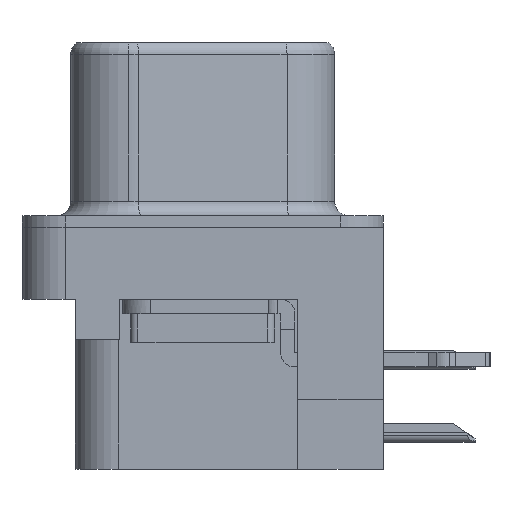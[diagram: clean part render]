
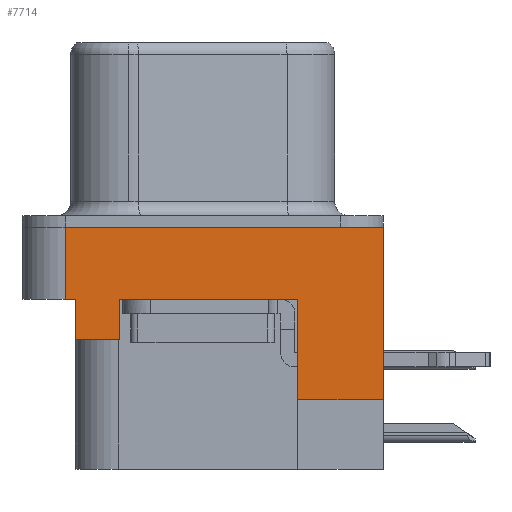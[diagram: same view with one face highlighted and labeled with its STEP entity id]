
A CAD part, left-side view. The second image highlights one B-rep face of the part: STEP entity #7714.
In plain terms, the highlighted planar face has unit normal (-1, 0, 0).
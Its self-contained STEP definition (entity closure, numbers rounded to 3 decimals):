
#115 = CARTESIAN_POINT ( 'NONE',  ( -3., -3.295, -6. ) ) ;
#613 = CARTESIAN_POINT ( 'NONE',  ( -3., 4.425, -3.9 ) ) ;
#843 = VECTOR ( 'NONE', #7435, 1000. ) ;
#917 = AXIS2_PLACEMENT_3D ( 'NONE', #3185, #8487, #19113 ) ;
#1014 = ORIENTED_EDGE ( 'NONE', *, *, #11626, .F. ) ;
#1609 = VECTOR ( 'NONE', #16953, 1000. ) ;
#1966 = VERTEX_POINT ( 'NONE', #12469 ) ;
#2138 = VERTEX_POINT ( 'NONE', #115 ) ;
#3038 = VERTEX_POINT ( 'NONE', #7005 ) ;
#3185 = CARTESIAN_POINT ( 'NONE',  ( -3., -6.275, -2.5 ) ) ;
#3425 = ORIENTED_EDGE ( 'NONE', *, *, #12761, .F. ) ;
#3819 = LINE ( 'NONE', #12870, #16233 ) ;
#4087 = DIRECTION ( 'NONE',  ( 0., 1., 0. ) ) ;
#4312 = ORIENTED_EDGE ( 'NONE', *, *, #11409, .T. ) ;
#4371 = VECTOR ( 'NONE', #13224, 1000. ) ;
#4519 = ORIENTED_EDGE ( 'NONE', *, *, #12701, .F. ) ;
#4573 = CARTESIAN_POINT ( 'NONE',  ( -3., -6.275, -2.5 ) ) ;
#5226 = ORIENTED_EDGE ( 'NONE', *, *, #11231, .F. ) ;
#5701 = CARTESIAN_POINT ( 'NONE',  ( -3., -3.295, -2.5 ) ) ;
#5718 = CARTESIAN_POINT ( 'NONE',  ( -3., 4.425, -3.9 ) ) ;
#6005 = FACE_OUTER_BOUND ( 'NONE', #9215, .T. ) ;
#6020 = CARTESIAN_POINT ( 'NONE',  ( -3., 4.775, 0. ) ) ;
#6402 = VERTEX_POINT ( 'NONE', #15309 ) ;
#6598 = EDGE_CURVE ( 'NONE', #18283, #12786, #11634, .T. ) ;
#6743 = ORIENTED_EDGE ( 'NONE', *, *, #13139, .F. ) ;
#6930 = CARTESIAN_POINT ( 'NONE',  ( -3., -6.275, 0. ) ) ;
#7005 = CARTESIAN_POINT ( 'NONE',  ( -3., -6.275, -6. ) ) ;
#7435 = DIRECTION ( 'NONE',  ( 0., 1., 0. ) ) ;
#7712 = ORIENTED_EDGE ( 'NONE', *, *, #9236, .F. ) ;
#7714 = ADVANCED_FACE ( 'NONE', ( #6005 ), #8132, .T. ) ;
#7829 = EDGE_CURVE ( 'NONE', #14547, #18283, #8804, .T. ) ;
#8132 = PLANE ( 'NONE',  #917 ) ;
#8487 = DIRECTION ( 'NONE',  ( -1., 0., 0. ) ) ;
#8702 = CARTESIAN_POINT ( 'NONE',  ( -3., 4.775, -2.5 ) ) ;
#8804 = LINE ( 'NONE', #19328, #16292 ) ;
#9070 = DIRECTION ( 'NONE',  ( 0., -1., 0. ) ) ;
#9215 = EDGE_LOOP ( 'NONE', ( #5226, #4312, #1014, #4519, #17532, #3425, #7712, #11055, #17895, #6743 ) ) ;
#9236 = EDGE_CURVE ( 'NONE', #14547, #11448, #13190, .T. ) ;
#9584 = LINE ( 'NONE', #16430, #843 ) ;
#9824 = DIRECTION ( 'NONE',  ( 0., -1., 0. ) ) ;
#9842 = CARTESIAN_POINT ( 'NONE',  ( -3., 2.895, -3.9 ) ) ;
#9978 = EDGE_CURVE ( 'NONE', #10033, #1966, #14787, .T. ) ;
#10033 = VERTEX_POINT ( 'NONE', #12123 ) ;
#10980 = LINE ( 'NONE', #6930, #14955 ) ;
#11055 = ORIENTED_EDGE ( 'NONE', *, *, #7829, .T. ) ;
#11231 = EDGE_CURVE ( 'NONE', #3038, #2138, #9584, .T. ) ;
#11409 = EDGE_CURVE ( 'NONE', #3038, #6402, #18351, .T. ) ;
#11448 = VERTEX_POINT ( 'NONE', #17078 ) ;
#11626 = EDGE_CURVE ( 'NONE', #11953, #6402, #10980, .T. ) ;
#11634 = LINE ( 'NONE', #20498, #15116 ) ;
#11804 = VECTOR ( 'NONE', #11911, 1000. ) ;
#11911 = DIRECTION ( 'NONE',  ( 0., 0., 1. ) ) ;
#11953 = VERTEX_POINT ( 'NONE', #6020 ) ;
#12123 = CARTESIAN_POINT ( 'NONE',  ( -3., 4.775, -2.5 ) ) ;
#12469 = CARTESIAN_POINT ( 'NONE',  ( -3., 4.425, -2.5 ) ) ;
#12701 = EDGE_CURVE ( 'NONE', #10033, #11953, #13218, .T. ) ;
#12761 = EDGE_CURVE ( 'NONE', #11448, #1966, #19454, .T. ) ;
#12786 = VERTEX_POINT ( 'NONE', #5701 ) ;
#12870 = CARTESIAN_POINT ( 'NONE',  ( -3., -3.295, -8.4 ) ) ;
#12903 = CARTESIAN_POINT ( 'NONE',  ( -3., 2.895, -2.5 ) ) ;
#13139 = EDGE_CURVE ( 'NONE', #2138, #12786, #3819, .T. ) ;
#13190 = LINE ( 'NONE', #5718, #16229 ) ;
#13218 = LINE ( 'NONE', #8702, #4371 ) ;
#13224 = DIRECTION ( 'NONE',  ( 0., 0., 1. ) ) ;
#14454 = DIRECTION ( 'NONE',  ( 0., -1., 0. ) ) ;
#14547 = VERTEX_POINT ( 'NONE', #9842 ) ;
#14691 = DIRECTION ( 'NONE',  ( 0., 0., 1. ) ) ;
#14787 = LINE ( 'NONE', #18092, #18898 ) ;
#14955 = VECTOR ( 'NONE', #14454, 1000. ) ;
#15116 = VECTOR ( 'NONE', #9824, 1000. ) ;
#15309 = CARTESIAN_POINT ( 'NONE',  ( -3., -6.275, 0. ) ) ;
#15859 = DIRECTION ( 'NONE',  ( 0., 0., 1. ) ) ;
#16229 = VECTOR ( 'NONE', #4087, 1000. ) ;
#16233 = VECTOR ( 'NONE', #15859, 1000. ) ;
#16292 = VECTOR ( 'NONE', #14691, 1000. ) ;
#16430 = CARTESIAN_POINT ( 'NONE',  ( -3., -6.495, -6. ) ) ;
#16953 = DIRECTION ( 'NONE',  ( 0., 0., 1. ) ) ;
#17078 = CARTESIAN_POINT ( 'NONE',  ( -3., 4.425, -3.9 ) ) ;
#17532 = ORIENTED_EDGE ( 'NONE', *, *, #9978, .T. ) ;
#17895 = ORIENTED_EDGE ( 'NONE', *, *, #6598, .T. ) ;
#18092 = CARTESIAN_POINT ( 'NONE',  ( -3., -6.275, -2.5 ) ) ;
#18283 = VERTEX_POINT ( 'NONE', #12903 ) ;
#18351 = LINE ( 'NONE', #4573, #1609 ) ;
#18898 = VECTOR ( 'NONE', #9070, 1000. ) ;
#19113 = DIRECTION ( 'NONE',  ( 0., 0., 1. ) ) ;
#19328 = CARTESIAN_POINT ( 'NONE',  ( -3., 2.895, -3.9 ) ) ;
#19454 = LINE ( 'NONE', #613, #11804 ) ;
#20498 = CARTESIAN_POINT ( 'NONE',  ( -3., -6.275, -2.5 ) ) ;
